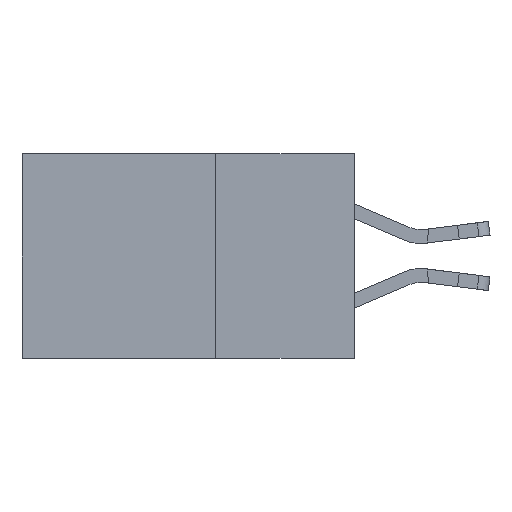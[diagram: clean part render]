
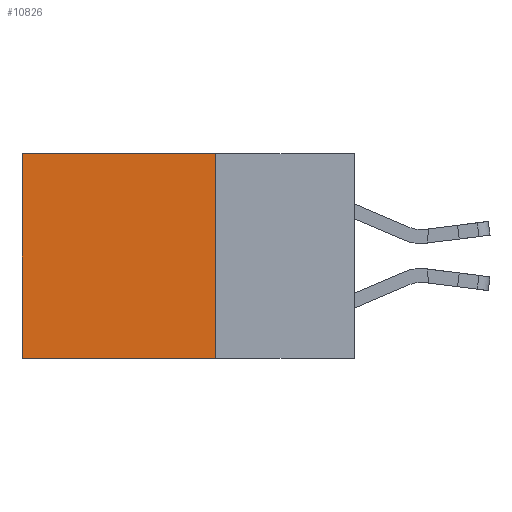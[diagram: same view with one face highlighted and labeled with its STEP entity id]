
A CAD part, left-side view. The second image highlights one B-rep face of the part: STEP entity #10826.
In plain terms, the highlighted planar face has unit normal (-1, 0, 0).
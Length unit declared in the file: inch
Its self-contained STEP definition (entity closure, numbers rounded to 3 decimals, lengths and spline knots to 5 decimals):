
#467 = DIRECTION ( 'NONE',  ( 1., 0., 0. ) ) ;
#2716 = CARTESIAN_POINT ( 'NONE',  ( 0.2615, 0.25, 0. ) ) ;
#2744 = CARTESIAN_POINT ( 'NONE',  ( 0.2615, 0.6, 0. ) ) ;
#2817 = ORIENTED_EDGE ( 'NONE', *, *, #15596, .T. ) ;
#4255 = VECTOR ( 'NONE', #15492, 39.37008 ) ;
#4575 = VECTOR ( 'NONE', #12350, 39.37008 ) ;
#4666 = CARTESIAN_POINT ( 'NONE',  ( 0.2615, 0.25, -0.37 ) ) ;
#5319 = CARTESIAN_POINT ( 'NONE',  ( 0.2615, 0.25, -0.37 ) ) ;
#5323 = LINE ( 'NONE', #20150, #4255 ) ;
#5332 = VERTEX_POINT ( 'NONE', #18053 ) ;
#7162 = CARTESIAN_POINT ( 'NONE',  ( 0.2615, 0.25, 0. ) ) ;
#8872 = VERTEX_POINT ( 'NONE', #2744 ) ;
#8888 = EDGE_CURVE ( 'NONE', #17871, #19547, #13256, .T. ) ;
#9887 = CARTESIAN_POINT ( 'NONE',  ( 0.2615, 0.25, -0.37 ) ) ;
#10180 = DIRECTION ( 'NONE',  ( 0., 0., -1. ) ) ;
#10463 = ORIENTED_EDGE ( 'NONE', *, *, #19156, .T. ) ;
#10826 = ADVANCED_FACE ( 'NONE', ( #11693 ), #15066, .F. ) ;
#11059 = VECTOR ( 'NONE', #18944, 39.37008 ) ;
#11693 = FACE_OUTER_BOUND ( 'NONE', #16771, .T. ) ;
#12350 = DIRECTION ( 'NONE',  ( 0., 1., 0. ) ) ;
#13256 = LINE ( 'NONE', #9887, #15274 ) ;
#14189 = CARTESIAN_POINT ( 'NONE',  ( 0.2615, 0.25, -0.37 ) ) ;
#14877 = DIRECTION ( 'NONE',  ( 0., 0., -1. ) ) ;
#15066 = PLANE ( 'NONE',  #17535 ) ;
#15274 = VECTOR ( 'NONE', #14877, 39.37008 ) ;
#15435 = ORIENTED_EDGE ( 'NONE', *, *, #8888, .F. ) ;
#15492 = DIRECTION ( 'NONE',  ( 0., 0., -1. ) ) ;
#15596 = EDGE_CURVE ( 'NONE', #17871, #8872, #17428, .T. ) ;
#16311 = ORIENTED_EDGE ( 'NONE', *, *, #18112, .F. ) ;
#16771 = EDGE_LOOP ( 'NONE', ( #10463, #16311, #15435, #2817 ) ) ;
#17428 = LINE ( 'NONE', #2716, #11059 ) ;
#17535 = AXIS2_PLACEMENT_3D ( 'NONE', #5319, #467, #10180 ) ;
#17871 = VERTEX_POINT ( 'NONE', #7162 ) ;
#18053 = CARTESIAN_POINT ( 'NONE',  ( 0.2615, 0.6, -0.37 ) ) ;
#18112 = EDGE_CURVE ( 'NONE', #19547, #5332, #19033, .T. ) ;
#18944 = DIRECTION ( 'NONE',  ( 0., 1., 0. ) ) ;
#19033 = LINE ( 'NONE', #14189, #4575 ) ;
#19156 = EDGE_CURVE ( 'NONE', #8872, #5332, #5323, .T. ) ;
#19547 = VERTEX_POINT ( 'NONE', #4666 ) ;
#20150 = CARTESIAN_POINT ( 'NONE',  ( 0.2615, 0.6, -0.37 ) ) ;
